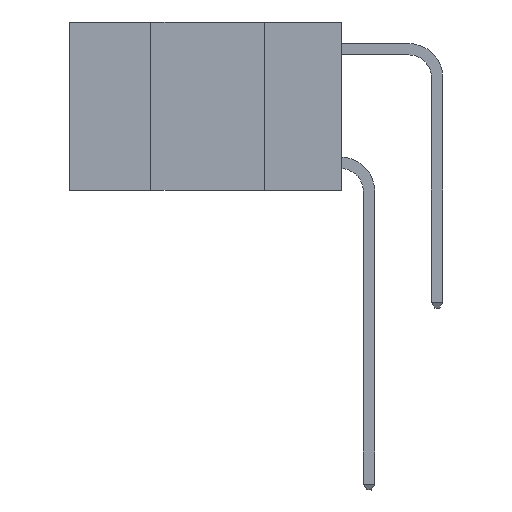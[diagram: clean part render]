
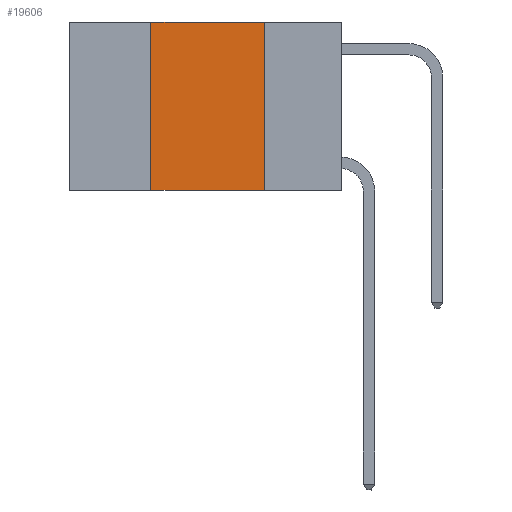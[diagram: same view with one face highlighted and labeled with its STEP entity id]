
A CAD part, left-side view. The second image highlights one B-rep face of the part: STEP entity #19606.
In plain terms, the highlighted planar face has unit normal (-1, 0, 0).
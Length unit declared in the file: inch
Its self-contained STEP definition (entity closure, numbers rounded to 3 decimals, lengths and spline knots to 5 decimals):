
#437 = CARTESIAN_POINT ( 'NONE',  ( 0., 0.17, -0.37 ) ) ;
#1452 = CARTESIAN_POINT ( 'NONE',  ( 0., 0.6, 0. ) ) ;
#1542 = FACE_OUTER_BOUND ( 'NONE', #21381, .T. ) ;
#1767 = LINE ( 'NONE', #8586, #23116 ) ;
#2326 = LINE ( 'NONE', #1452, #5522 ) ;
#2380 = ORIENTED_EDGE ( 'NONE', *, *, #18289, .F. ) ;
#2503 = CARTESIAN_POINT ( 'NONE',  ( 0., 0.42, -0.37 ) ) ;
#3226 = DIRECTION ( 'NONE',  ( 1., 0., 0. ) ) ;
#3883 = AXIS2_PLACEMENT_3D ( 'NONE', #9528, #3226, #25923 ) ;
#4007 = VERTEX_POINT ( 'NONE', #437 ) ;
#5522 = VECTOR ( 'NONE', #25975, 39.37008 ) ;
#5837 = CARTESIAN_POINT ( 'NONE',  ( 0., 0.42, 0. ) ) ;
#7512 = PLANE ( 'NONE',  #3883 ) ;
#7748 = EDGE_CURVE ( 'NONE', #25866, #4007, #1767, .T. ) ;
#8586 = CARTESIAN_POINT ( 'NONE',  ( 0., 0.6, -0.37 ) ) ;
#9528 = CARTESIAN_POINT ( 'NONE',  ( 0., 0.6, 0. ) ) ;
#9753 = EDGE_CURVE ( 'NONE', #26727, #4007, #14092, .T. ) ;
#10224 = VERTEX_POINT ( 'NONE', #5837 ) ;
#11221 = ORIENTED_EDGE ( 'NONE', *, *, #9753, .F. ) ;
#11435 = CARTESIAN_POINT ( 'NONE',  ( 0., 0.42, 0. ) ) ;
#14092 = LINE ( 'NONE', #16546, #18288 ) ;
#14439 = DIRECTION ( 'NONE',  ( 0., 0., -1. ) ) ;
#15658 = DIRECTION ( 'NONE',  ( 0., 0., 1. ) ) ;
#16466 = EDGE_CURVE ( 'NONE', #10224, #26727, #2326, .T. ) ;
#16546 = CARTESIAN_POINT ( 'NONE',  ( 0., 0.17, 0. ) ) ;
#18288 = VECTOR ( 'NONE', #14439, 39.37008 ) ;
#18289 = EDGE_CURVE ( 'NONE', #25866, #10224, #26176, .T. ) ;
#18479 = ORIENTED_EDGE ( 'NONE', *, *, #7748, .T. ) ;
#19606 = ADVANCED_FACE ( 'NONE', ( #1542 ), #7512, .F. ) ;
#20626 = VECTOR ( 'NONE', #15658, 39.37008 ) ;
#21381 = EDGE_LOOP ( 'NONE', ( #11221, #22599, #2380, #18479 ) ) ;
#22599 = ORIENTED_EDGE ( 'NONE', *, *, #16466, .F. ) ;
#23116 = VECTOR ( 'NONE', #24815, 39.37008 ) ;
#24815 = DIRECTION ( 'NONE',  ( 0., -1., 0. ) ) ;
#25312 = CARTESIAN_POINT ( 'NONE',  ( 0., 0.17, 0. ) ) ;
#25866 = VERTEX_POINT ( 'NONE', #2503 ) ;
#25923 = DIRECTION ( 'NONE',  ( 0., 0., -1. ) ) ;
#25975 = DIRECTION ( 'NONE',  ( 0., -1., 0. ) ) ;
#26176 = LINE ( 'NONE', #11435, #20626 ) ;
#26727 = VERTEX_POINT ( 'NONE', #25312 ) ;
